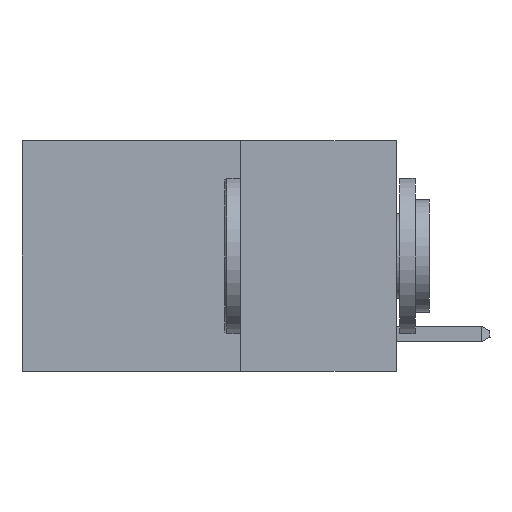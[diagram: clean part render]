
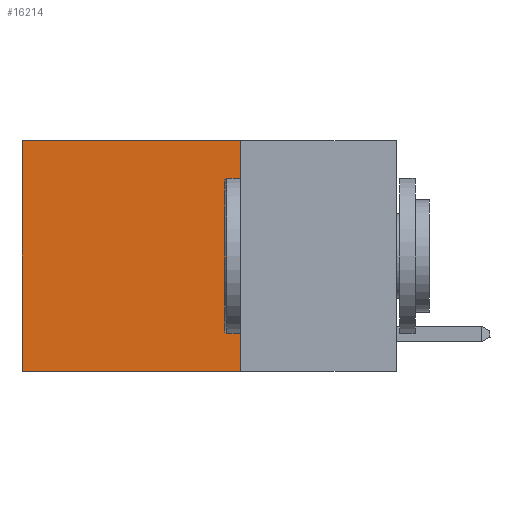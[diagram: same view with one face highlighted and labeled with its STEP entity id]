
A CAD part, left-side view. The second image highlights one B-rep face of the part: STEP entity #16214.
In plain terms, the highlighted planar face has unit normal (-1, 0, 0).
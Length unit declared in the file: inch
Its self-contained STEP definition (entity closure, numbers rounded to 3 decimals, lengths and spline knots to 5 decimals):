
#77 = CARTESIAN_POINT ( 'NONE',  ( 0.2625, 0.6, 0. ) ) ;
#128 = VERTEX_POINT ( 'NONE', #9094 ) ;
#560 = EDGE_CURVE ( 'NONE', #128, #21915, #2952, .T. ) ;
#2648 = LINE ( 'NONE', #9565, #15871 ) ;
#2952 = LINE ( 'NONE', #5006, #15639 ) ;
#3664 = DIRECTION ( 'NONE',  ( 0., 0., -1. ) ) ;
#3704 = ORIENTED_EDGE ( 'NONE', *, *, #12699, .F. ) ;
#4094 = CARTESIAN_POINT ( 'NONE',  ( 0.2625, 0.25, 0. ) ) ;
#4615 = FACE_OUTER_BOUND ( 'NONE', #7095, .T. ) ;
#5006 = CARTESIAN_POINT ( 'NONE',  ( 0.2625, 0.25, 0. ) ) ;
#5600 = CARTESIAN_POINT ( 'NONE',  ( 0.2625, 0.25, -0.37 ) ) ;
#5621 = LINE ( 'NONE', #4094, #18293 ) ;
#7095 = EDGE_LOOP ( 'NONE', ( #14806, #3704, #9874, #15173 ) ) ;
#8345 = VECTOR ( 'NONE', #3664, 39.37008 ) ;
#9094 = CARTESIAN_POINT ( 'NONE',  ( 0.2625, 0.25, 0. ) ) ;
#9565 = CARTESIAN_POINT ( 'NONE',  ( 0.2625, 0.25, -0.37 ) ) ;
#9874 = ORIENTED_EDGE ( 'NONE', *, *, #560, .F. ) ;
#10002 = DIRECTION ( 'NONE',  ( 1., 0., 0. ) ) ;
#11294 = DIRECTION ( 'NONE',  ( 0., 1., 0. ) ) ;
#11650 = CARTESIAN_POINT ( 'NONE',  ( 0.2625, 0.25, 0. ) ) ;
#12201 = CARTESIAN_POINT ( 'NONE',  ( 0.2625, 0.6, -0.37 ) ) ;
#12699 = EDGE_CURVE ( 'NONE', #21915, #17064, #2648, .T. ) ;
#12706 = DIRECTION ( 'NONE',  ( 0., 1., 0. ) ) ;
#12926 = LINE ( 'NONE', #77, #8345 ) ;
#14806 = ORIENTED_EDGE ( 'NONE', *, *, #19302, .T. ) ;
#15173 = ORIENTED_EDGE ( 'NONE', *, *, #19504, .T. ) ;
#15639 = VECTOR ( 'NONE', #15725, 39.37008 ) ;
#15725 = DIRECTION ( 'NONE',  ( 0., 0., -1. ) ) ;
#15871 = VECTOR ( 'NONE', #11294, 39.37008 ) ;
#16214 = ADVANCED_FACE ( 'NONE', ( #4615 ), #20276, .F. ) ;
#17064 = VERTEX_POINT ( 'NONE', #12201 ) ;
#17204 = CARTESIAN_POINT ( 'NONE',  ( 0.2625, 0.6, 0. ) ) ;
#18293 = VECTOR ( 'NONE', #12706, 39.37008 ) ;
#19302 = EDGE_CURVE ( 'NONE', #21763, #17064, #12926, .T. ) ;
#19504 = EDGE_CURVE ( 'NONE', #128, #21763, #5621, .T. ) ;
#19912 = AXIS2_PLACEMENT_3D ( 'NONE', #11650, #10002, #22021 ) ;
#20276 = PLANE ( 'NONE',  #19912 ) ;
#21763 = VERTEX_POINT ( 'NONE', #17204 ) ;
#21915 = VERTEX_POINT ( 'NONE', #5600 ) ;
#22021 = DIRECTION ( 'NONE',  ( 0., 0., -1. ) ) ;
